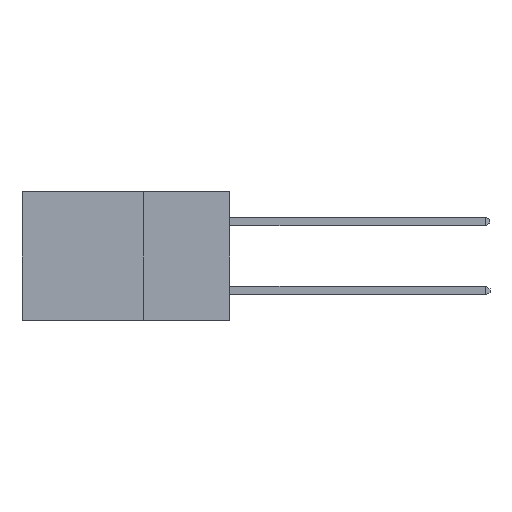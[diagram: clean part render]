
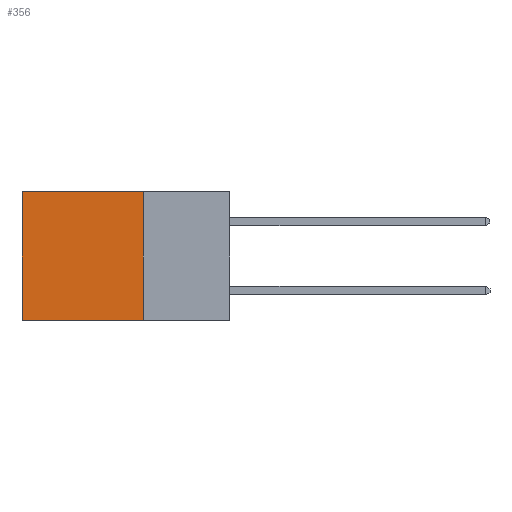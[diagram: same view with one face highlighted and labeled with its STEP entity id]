
A CAD part, left-side view. The second image highlights one B-rep face of the part: STEP entity #356.
In plain terms, the highlighted planar face has unit normal (-1, 0, 0).
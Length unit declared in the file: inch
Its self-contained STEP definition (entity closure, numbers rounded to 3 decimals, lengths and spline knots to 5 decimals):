
#297 = DIRECTION ( 'NONE',  ( 0., 1., 0. ) ) ;
#319 = FACE_OUTER_BOUND ( 'NONE', #10375, .T. ) ;
#356 = ADVANCED_FACE ( 'NONE', ( #319 ), #11896, .F. ) ;
#373 = CARTESIAN_POINT ( 'NONE',  ( 0.2615, 0.25, -0.37 ) ) ;
#559 = VECTOR ( 'NONE', #7576, 39.37008 ) ;
#1810 = EDGE_CURVE ( 'NONE', #4456, #10543, #6737, .T. ) ;
#1954 = LINE ( 'NONE', #4014, #6600 ) ;
#2309 = VERTEX_POINT ( 'NONE', #4369 ) ;
#2606 = AXIS2_PLACEMENT_3D ( 'NONE', #6998, #4888, #7596 ) ;
#2646 = CARTESIAN_POINT ( 'NONE',  ( 0.2615, 0.6, 0. ) ) ;
#3580 = CARTESIAN_POINT ( 'NONE',  ( 0.2615, 0.6, -0.37 ) ) ;
#3676 = DIRECTION ( 'NONE',  ( 0., 0., -1. ) ) ;
#4002 = DIRECTION ( 'NONE',  ( 0., 0., -1. ) ) ;
#4014 = CARTESIAN_POINT ( 'NONE',  ( 0.2615, 0.25, -0.37 ) ) ;
#4308 = VECTOR ( 'NONE', #3676, 39.37008 ) ;
#4369 = CARTESIAN_POINT ( 'NONE',  ( 0.2615, 0.25, 0. ) ) ;
#4456 = VERTEX_POINT ( 'NONE', #9889 ) ;
#4888 = DIRECTION ( 'NONE',  ( 1., 0., 0. ) ) ;
#5648 = ORIENTED_EDGE ( 'NONE', *, *, #8449, .T. ) ;
#5778 = EDGE_CURVE ( 'NONE', #2309, #4456, #1954, .T. ) ;
#5942 = ORIENTED_EDGE ( 'NONE', *, *, #1810, .F. ) ;
#6600 = VECTOR ( 'NONE', #4002, 39.37008 ) ;
#6675 = ORIENTED_EDGE ( 'NONE', *, *, #5778, .F. ) ;
#6737 = LINE ( 'NONE', #373, #7033 ) ;
#6998 = CARTESIAN_POINT ( 'NONE',  ( 0.2615, 0.25, -0.37 ) ) ;
#7033 = VECTOR ( 'NONE', #297, 39.37008 ) ;
#7468 = EDGE_CURVE ( 'NONE', #2309, #11053, #8035, .T. ) ;
#7576 = DIRECTION ( 'NONE',  ( 0., 1., 0. ) ) ;
#7596 = DIRECTION ( 'NONE',  ( 0., 0., -1. ) ) ;
#7618 = CARTESIAN_POINT ( 'NONE',  ( 0.2615, 0.25, 0. ) ) ;
#8035 = LINE ( 'NONE', #7618, #559 ) ;
#8058 = CARTESIAN_POINT ( 'NONE',  ( 0.2615, 0.6, -0.37 ) ) ;
#8449 = EDGE_CURVE ( 'NONE', #11053, #10543, #9296, .T. ) ;
#9126 = ORIENTED_EDGE ( 'NONE', *, *, #7468, .T. ) ;
#9296 = LINE ( 'NONE', #3580, #4308 ) ;
#9889 = CARTESIAN_POINT ( 'NONE',  ( 0.2615, 0.25, -0.37 ) ) ;
#10375 = EDGE_LOOP ( 'NONE', ( #5648, #5942, #6675, #9126 ) ) ;
#10543 = VERTEX_POINT ( 'NONE', #8058 ) ;
#11053 = VERTEX_POINT ( 'NONE', #2646 ) ;
#11896 = PLANE ( 'NONE',  #2606 ) ;
